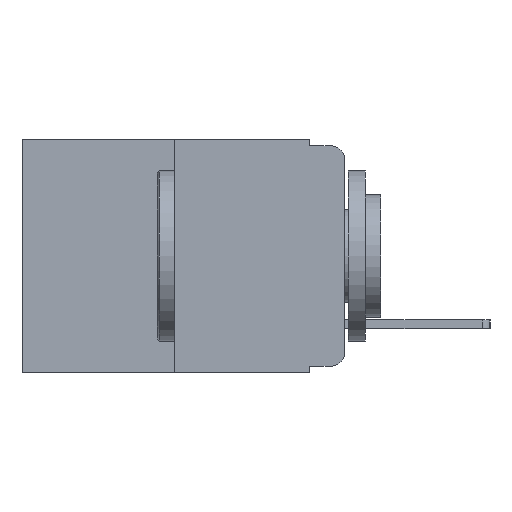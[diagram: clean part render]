
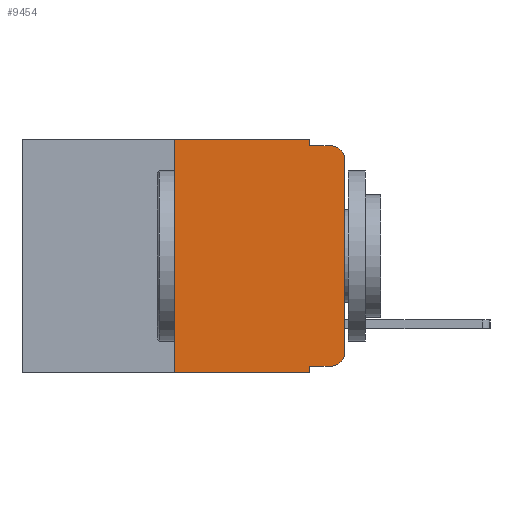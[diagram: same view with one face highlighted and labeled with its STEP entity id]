
A CAD part, left-side view. The second image highlights one B-rep face of the part: STEP entity #9454.
In plain terms, the highlighted planar face has unit normal (-1, 0, 0).
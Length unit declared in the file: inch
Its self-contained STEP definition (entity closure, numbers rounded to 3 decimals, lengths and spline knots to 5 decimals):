
#294 = EDGE_CURVE ( 'NONE', #16665, #5448, #2248, .T. ) ;
#338 = VERTEX_POINT ( 'NONE', #12634 ) ;
#420 = EDGE_CURVE ( 'NONE', #17254, #11201, #4449, .T. ) ;
#850 = AXIS2_PLACEMENT_3D ( 'NONE', #7511, #4272, #18347 ) ;
#925 = VECTOR ( 'NONE', #7756, 39.37008 ) ;
#961 = LINE ( 'NONE', #17788, #16432 ) ;
#1199 = VERTEX_POINT ( 'NONE', #15815 ) ;
#1206 = LINE ( 'NONE', #5456, #12468 ) ;
#1524 = EDGE_CURVE ( 'NONE', #4537, #18439, #3692, .T. ) ;
#2248 = LINE ( 'NONE', #17688, #11834 ) ;
#2525 = VECTOR ( 'NONE', #12300, 39.37008 ) ;
#3692 = LINE ( 'NONE', #5071, #18781 ) ;
#3754 = VECTOR ( 'NONE', #9307, 39.37008 ) ;
#3788 = CARTESIAN_POINT ( 'NONE',  ( 0., 0., -0.313 ) ) ;
#4170 = ORIENTED_EDGE ( 'NONE', *, *, #294, .F. ) ;
#4272 = DIRECTION ( 'NONE',  ( -1., 0., 0. ) ) ;
#4281 = CARTESIAN_POINT ( 'NONE',  ( 0., 0.473, -0.343 ) ) ;
#4449 = CIRCLE ( 'NONE', #850, 0.02 ) ;
#4537 = VERTEX_POINT ( 'NONE', #11036 ) ;
#4897 = ORIENTED_EDGE ( 'NONE', *, *, #5086, .T. ) ;
#5071 = CARTESIAN_POINT ( 'NONE',  ( 0., 0.25, 0. ) ) ;
#5086 = EDGE_CURVE ( 'NONE', #1199, #5279, #5739, .T. ) ;
#5279 = VERTEX_POINT ( 'NONE', #3788 ) ;
#5448 = VERTEX_POINT ( 'NONE', #10415 ) ;
#5456 = CARTESIAN_POINT ( 'NONE',  ( 0., 0., 0. ) ) ;
#5739 = CIRCLE ( 'NONE', #6359, 0.02 ) ;
#5992 = EDGE_CURVE ( 'NONE', #5448, #11201, #7850, .T. ) ;
#6284 = CARTESIAN_POINT ( 'NONE',  ( 0., 0.051, 0. ) ) ;
#6359 = AXIS2_PLACEMENT_3D ( 'NONE', #15205, #6393, #16599 ) ;
#6393 = DIRECTION ( 'NONE',  ( -1., 0., 0. ) ) ;
#6617 = DIRECTION ( 'NONE',  ( 0., 0., -1. ) ) ;
#6667 = LINE ( 'NONE', #19164, #2525 ) ;
#6861 = EDGE_CURVE ( 'NONE', #4537, #338, #10903, .T. ) ;
#7511 = CARTESIAN_POINT ( 'NONE',  ( 0., 0.02, -0.03 ) ) ;
#7756 = DIRECTION ( 'NONE',  ( 0., -1., 0. ) ) ;
#7850 = LINE ( 'NONE', #17865, #3754 ) ;
#8024 = CARTESIAN_POINT ( 'NONE',  ( 0., 0.02, -0.01 ) ) ;
#8418 = EDGE_CURVE ( 'NONE', #18439, #16665, #16851, .T. ) ;
#9282 = CARTESIAN_POINT ( 'NONE',  ( 0., 0.473, 0. ) ) ;
#9307 = DIRECTION ( 'NONE',  ( 0., -1., 0. ) ) ;
#9454 = ADVANCED_FACE ( 'NONE', ( #10084 ), #17271, .F. ) ;
#10084 = FACE_OUTER_BOUND ( 'NONE', #14233, .T. ) ;
#10103 = DIRECTION ( 'NONE',  ( 0., 0., 1. ) ) ;
#10159 = DIRECTION ( 'NONE',  ( 0., 0., -1. ) ) ;
#10415 = CARTESIAN_POINT ( 'NONE',  ( 0., 0.051, -0.01 ) ) ;
#10903 = LINE ( 'NONE', #4281, #14264 ) ;
#11036 = CARTESIAN_POINT ( 'NONE',  ( 0., 0.25, -0.343 ) ) ;
#11201 = VERTEX_POINT ( 'NONE', #8024 ) ;
#11834 = VECTOR ( 'NONE', #6617, 39.37008 ) ;
#11876 = VERTEX_POINT ( 'NONE', #17954 ) ;
#12039 = ORIENTED_EDGE ( 'NONE', *, *, #18175, .T. ) ;
#12300 = DIRECTION ( 'NONE',  ( 0., 0., -1. ) ) ;
#12468 = VECTOR ( 'NONE', #12954, 39.37008 ) ;
#12567 = EDGE_CURVE ( 'NONE', #11876, #338, #6667, .T. ) ;
#12634 = CARTESIAN_POINT ( 'NONE',  ( 0., 0.051, -0.343 ) ) ;
#12954 = DIRECTION ( 'NONE',  ( 0., 0., 1. ) ) ;
#14233 = EDGE_LOOP ( 'NONE', ( #17942, #15139, #19215, #4170, #16445, #16890, #17325, #18161, #12039, #4897 ) ) ;
#14264 = VECTOR ( 'NONE', #14735, 39.37008 ) ;
#14454 = CARTESIAN_POINT ( 'NONE',  ( 0., 0.473, 0. ) ) ;
#14735 = DIRECTION ( 'NONE',  ( 0., -1., 0. ) ) ;
#15139 = ORIENTED_EDGE ( 'NONE', *, *, #420, .T. ) ;
#15205 = CARTESIAN_POINT ( 'NONE',  ( 0., 0.02, -0.313 ) ) ;
#15815 = CARTESIAN_POINT ( 'NONE',  ( 0., 0.02, -0.333 ) ) ;
#16432 = VECTOR ( 'NONE', #16462, 39.37008 ) ;
#16445 = ORIENTED_EDGE ( 'NONE', *, *, #8418, .F. ) ;
#16462 = DIRECTION ( 'NONE',  ( 0., -1., 0. ) ) ;
#16599 = DIRECTION ( 'NONE',  ( 0., 0., -1. ) ) ;
#16665 = VERTEX_POINT ( 'NONE', #6284 ) ;
#16851 = LINE ( 'NONE', #9282, #925 ) ;
#16890 = ORIENTED_EDGE ( 'NONE', *, *, #1524, .F. ) ;
#17254 = VERTEX_POINT ( 'NONE', #18872 ) ;
#17271 = PLANE ( 'NONE',  #18650 ) ;
#17325 = ORIENTED_EDGE ( 'NONE', *, *, #6861, .T. ) ;
#17688 = CARTESIAN_POINT ( 'NONE',  ( 0., 0.051, 0. ) ) ;
#17788 = CARTESIAN_POINT ( 'NONE',  ( 0., 0.051, -0.333 ) ) ;
#17865 = CARTESIAN_POINT ( 'NONE',  ( 0., 0.051, -0.01 ) ) ;
#17942 = ORIENTED_EDGE ( 'NONE', *, *, #18468, .T. ) ;
#17954 = CARTESIAN_POINT ( 'NONE',  ( 0., 0.051, -0.333 ) ) ;
#18161 = ORIENTED_EDGE ( 'NONE', *, *, #12567, .F. ) ;
#18175 = EDGE_CURVE ( 'NONE', #11876, #1199, #961, .T. ) ;
#18347 = DIRECTION ( 'NONE',  ( 0., 0., -1. ) ) ;
#18439 = VERTEX_POINT ( 'NONE', #18493 ) ;
#18468 = EDGE_CURVE ( 'NONE', #5279, #17254, #1206, .T. ) ;
#18493 = CARTESIAN_POINT ( 'NONE',  ( 0., 0.25, 0. ) ) ;
#18624 = DIRECTION ( 'NONE',  ( 1., 0., 0. ) ) ;
#18650 = AXIS2_PLACEMENT_3D ( 'NONE', #14454, #18624, #10159 ) ;
#18781 = VECTOR ( 'NONE', #10103, 39.37008 ) ;
#18872 = CARTESIAN_POINT ( 'NONE',  ( 0., 0., -0.03 ) ) ;
#19164 = CARTESIAN_POINT ( 'NONE',  ( 0., 0.051, 0. ) ) ;
#19215 = ORIENTED_EDGE ( 'NONE', *, *, #5992, .F. ) ;
